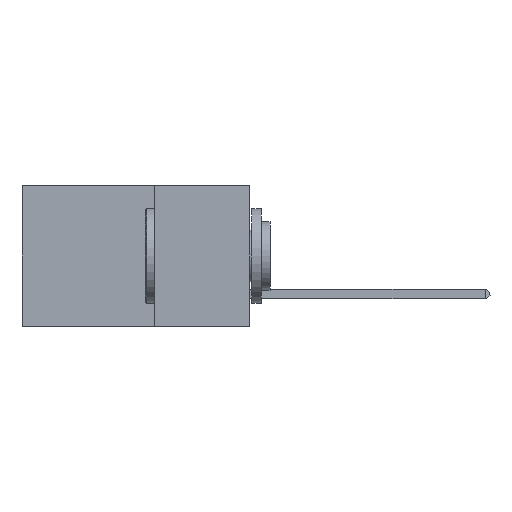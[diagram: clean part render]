
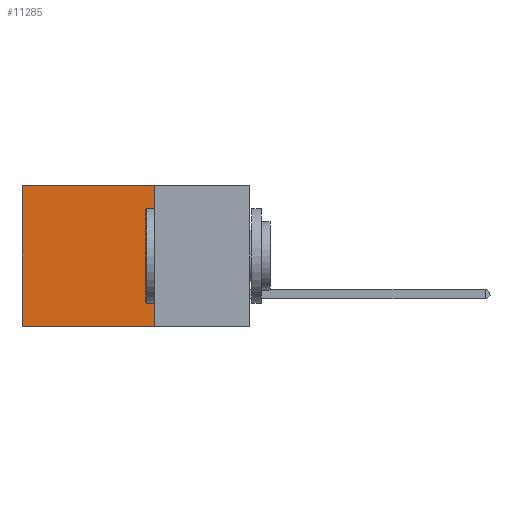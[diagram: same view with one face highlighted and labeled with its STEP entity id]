
A CAD part, left-side view. The second image highlights one B-rep face of the part: STEP entity #11285.
In plain terms, the highlighted planar face has unit normal (-1, 0, 0).
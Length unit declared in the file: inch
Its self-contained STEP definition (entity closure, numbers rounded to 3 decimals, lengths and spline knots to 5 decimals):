
#244 = DIRECTION ( 'NONE',  ( 0., 1., 0. ) ) ;
#446 = DIRECTION ( 'NONE',  ( 0., 1., 0. ) ) ;
#629 = ORIENTED_EDGE ( 'NONE', *, *, #11853, .F. ) ;
#1899 = EDGE_CURVE ( 'NONE', #12456, #9507, #13950, .T. ) ;
#4079 = CARTESIAN_POINT ( 'NONE',  ( 0.2875, 0.25, -0.37 ) ) ;
#4110 = FACE_OUTER_BOUND ( 'NONE', #9043, .T. ) ;
#4696 = CARTESIAN_POINT ( 'NONE',  ( 0.2875, 0.6, -0.37 ) ) ;
#4987 = AXIS2_PLACEMENT_3D ( 'NONE', #14342, #6264, #12070 ) ;
#5635 = VECTOR ( 'NONE', #14372, 39.37008 ) ;
#5888 = DIRECTION ( 'NONE',  ( 0., 0., -1. ) ) ;
#6160 = VECTOR ( 'NONE', #244, 39.37008 ) ;
#6264 = DIRECTION ( 'NONE',  ( 1., 0., 0. ) ) ;
#6398 = VERTEX_POINT ( 'NONE', #4696 ) ;
#7438 = LINE ( 'NONE', #9442, #14850 ) ;
#8612 = EDGE_CURVE ( 'NONE', #9507, #6398, #7438, .T. ) ;
#9043 = EDGE_LOOP ( 'NONE', ( #14638, #13858, #629, #10415 ) ) ;
#9275 = LINE ( 'NONE', #9682, #5635 ) ;
#9442 = CARTESIAN_POINT ( 'NONE',  ( 0.2875, 0.6, 0. ) ) ;
#9507 = VERTEX_POINT ( 'NONE', #13672 ) ;
#9682 = CARTESIAN_POINT ( 'NONE',  ( 0.2875, 0.25, 0. ) ) ;
#9870 = CARTESIAN_POINT ( 'NONE',  ( 0.2875, 0.25, 0. ) ) ;
#9880 = EDGE_CURVE ( 'NONE', #11269, #6398, #13745, .T. ) ;
#10415 = ORIENTED_EDGE ( 'NONE', *, *, #1899, .T. ) ;
#11020 = PLANE ( 'NONE',  #4987 ) ;
#11249 = VECTOR ( 'NONE', #446, 39.37008 ) ;
#11269 = VERTEX_POINT ( 'NONE', #4079 ) ;
#11285 = ADVANCED_FACE ( 'NONE', ( #4110 ), #11020, .F. ) ;
#11853 = EDGE_CURVE ( 'NONE', #12456, #11269, #9275, .T. ) ;
#11863 = CARTESIAN_POINT ( 'NONE',  ( 0.2875, 0.25, 0. ) ) ;
#12070 = DIRECTION ( 'NONE',  ( 0., 0., -1. ) ) ;
#12456 = VERTEX_POINT ( 'NONE', #9870 ) ;
#12701 = CARTESIAN_POINT ( 'NONE',  ( 0.2875, 0.25, -0.37 ) ) ;
#13672 = CARTESIAN_POINT ( 'NONE',  ( 0.2875, 0.6, 0. ) ) ;
#13745 = LINE ( 'NONE', #12701, #6160 ) ;
#13858 = ORIENTED_EDGE ( 'NONE', *, *, #9880, .F. ) ;
#13950 = LINE ( 'NONE', #11863, #11249 ) ;
#14342 = CARTESIAN_POINT ( 'NONE',  ( 0.2875, 0.25, 0. ) ) ;
#14372 = DIRECTION ( 'NONE',  ( 0., 0., -1. ) ) ;
#14638 = ORIENTED_EDGE ( 'NONE', *, *, #8612, .T. ) ;
#14850 = VECTOR ( 'NONE', #5888, 39.37008 ) ;
